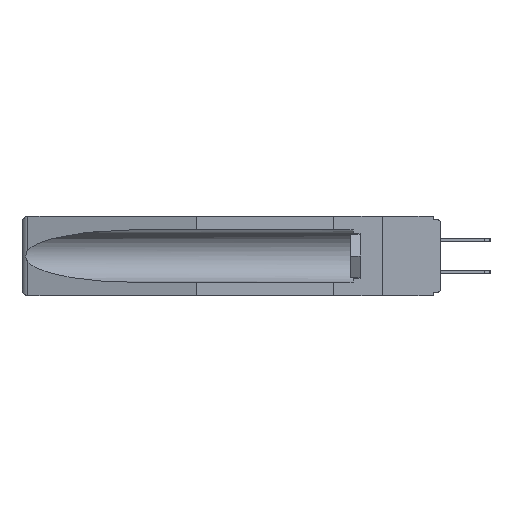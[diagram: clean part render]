
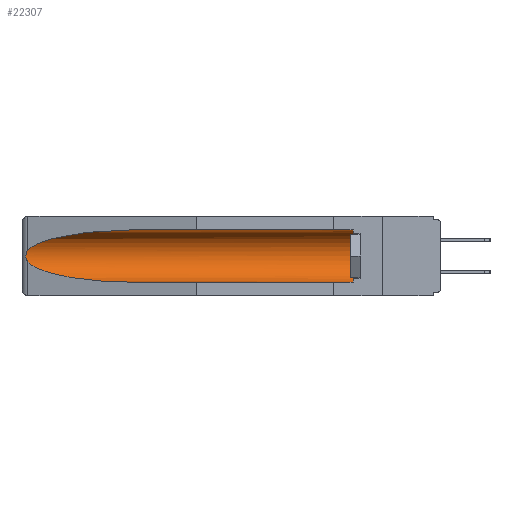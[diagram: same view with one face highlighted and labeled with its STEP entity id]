
A CAD part, left-side view. The second image highlights one B-rep face of the part: STEP entity #22307.
In plain terms, the highlighted cylindrical face has radius 2.857 mm (diameter 5.715 mm), a partial arc.
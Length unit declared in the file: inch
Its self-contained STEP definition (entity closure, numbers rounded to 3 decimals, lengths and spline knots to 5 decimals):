
#1272 = CARTESIAN_POINT ( 'NONE',  ( 0.25451, 1.48313, -0.09465 ) ) ;
#1772 = EDGE_CURVE ( 'NONE', #12204, #23187, #22237, .T. ) ;
#1898 = CARTESIAN_POINT ( 'NONE',  ( 0.26537, 1.52718, -0.14972 ) ) ;
#2437 = VERTEX_POINT ( 'NONE', #14347 ) ;
#3935 = CYLINDRICAL_SURFACE ( 'NONE', #19691, 0.1125 ) ;
#4100 = CARTESIAN_POINT ( 'NONE',  ( 0.2675, 1.53308, -0.17534 ) ) ;
#4671 = VERTEX_POINT ( 'NONE', #19808 ) ;
#5246 = CARTESIAN_POINT ( 'NONE',  ( 0.155, 0.126, -0.284 ) ) ;
#5372 =( BOUNDED_CURVE ( )  B_SPLINE_CURVE ( 3, ( #25111, #15462, #1272, #17284 ),
 .UNSPECIFIED., .F., .F. ) 
 B_SPLINE_CURVE_WITH_KNOTS ( ( 4, 4 ),
 ( 4.71239, 6.08839 ),
 .UNSPECIFIED. ) 
 CURVE ( )  GEOMETRIC_REPRESENTATION_ITEM ( )  RATIONAL_B_SPLINE_CURVE ( ( 1., 0.848, 0.848, 1. ) ) 
 REPRESENTATION_ITEM ( '' )  );
#5469 = VECTOR ( 'NONE', #18364, 39.37008 ) ;
#6264 = DIRECTION ( 'NONE',  ( 0., 0., 1. ) ) ;
#7159 = CARTESIAN_POINT ( 'NONE',  ( 0.26537, 1.52718, -0.19328 ) ) ;
#7236 = B_SPLINE_CURVE_WITH_KNOTS ( 'NONE', 3,
 ( #12720, #18549, #12638, #12551, #15929, #4100, #8487, #8741, #22394, #10460 ),
 .UNSPECIFIED., .F., .F.,
 ( 4, 2, 2, 2, 4 ),
 ( 0., 0.00029, 0.00058, 0.00087, 0.00117 ),
 .UNSPECIFIED. ) ;
#7256 = ORIENTED_EDGE ( 'NONE', *, *, #1772, .T. ) ;
#7600 = CARTESIAN_POINT ( 'NONE',  ( 0.155, 1.07973, -0.284 ) ) ;
#7628 = CARTESIAN_POINT ( 'NONE',  ( 0.155, -0.30754, -0.1715 ) ) ;
#7935 = VERTEX_POINT ( 'NONE', #5246 ) ;
#8487 = CARTESIAN_POINT ( 'NONE',  ( 0.2673, 1.53269, -0.17917 ) ) ;
#8741 = CARTESIAN_POINT ( 'NONE',  ( 0.26655, 1.53094, -0.18657 ) ) ;
#8783 = CARTESIAN_POINT ( 'NONE',  ( 0.26537, 1.52718, -0.19328 ) ) ;
#9243 = VECTOR ( 'NONE', #23481, 39.37008 ) ;
#9621 = DIRECTION ( 'NONE',  ( 0., 0., 1. ) ) ;
#10022 = EDGE_LOOP ( 'NONE', ( #16027, #10318, #7256, #18476, #14307, #12264 ) ) ;
#10318 = ORIENTED_EDGE ( 'NONE', *, *, #20927, .T. ) ;
#10460 = CARTESIAN_POINT ( 'NONE',  ( 0.26537, 1.52718, -0.19328 ) ) ;
#10995 = CARTESIAN_POINT ( 'NONE',  ( 0.155, 1.07973, -0.284 ) ) ;
#11872 = DIRECTION ( 'NONE',  ( 0., -1., 0. ) ) ;
#12204 = VERTEX_POINT ( 'NONE', #7159 ) ;
#12264 = ORIENTED_EDGE ( 'NONE', *, *, #15614, .T. ) ;
#12287 = CARTESIAN_POINT ( 'NONE',  ( 0.155, -0.30754, -0.059 ) ) ;
#12332 = EDGE_CURVE ( 'NONE', #7935, #4671, #13960, .T. ) ;
#12551 = CARTESIAN_POINT ( 'NONE',  ( 0.2673, 1.5327, -0.16383 ) ) ;
#12628 = EDGE_CURVE ( 'NONE', #2437, #24193, #5372, .T. ) ;
#12638 = CARTESIAN_POINT ( 'NONE',  ( 0.26654, 1.53092, -0.15636 ) ) ;
#12720 = CARTESIAN_POINT ( 'NONE',  ( 0.26537, 1.52718, -0.14972 ) ) ;
#13244 = DIRECTION ( 'NONE',  ( 0., 1., 0. ) ) ;
#13813 = FACE_OUTER_BOUND ( 'NONE', #10022, .T. ) ;
#13896 = LINE ( 'NONE', #21568, #9243 ) ;
#13960 = CIRCLE ( 'NONE', #17753, 0.1125 ) ;
#14307 = ORIENTED_EDGE ( 'NONE', *, *, #12332, .T. ) ;
#14347 = CARTESIAN_POINT ( 'NONE',  ( 0.155, 1.07973, -0.059 ) ) ;
#15462 = CARTESIAN_POINT ( 'NONE',  ( 0.21114, 1.30732, -0.059 ) ) ;
#15614 = EDGE_CURVE ( 'NONE', #4671, #2437, #25646, .T. ) ;
#15929 = CARTESIAN_POINT ( 'NONE',  ( 0.2675, 1.53308, -0.16763 ) ) ;
#16027 = ORIENTED_EDGE ( 'NONE', *, *, #12628, .T. ) ;
#16829 = CARTESIAN_POINT ( 'NONE',  ( 0.25451, 1.48313, -0.24835 ) ) ;
#17284 = CARTESIAN_POINT ( 'NONE',  ( 0.26537, 1.52718, -0.14972 ) ) ;
#17753 = AXIS2_PLACEMENT_3D ( 'NONE', #23770, #11872, #6264 ) ;
#18364 = DIRECTION ( 'NONE',  ( 0., 1., 0. ) ) ;
#18476 = ORIENTED_EDGE ( 'NONE', *, *, #24219, .F. ) ;
#18549 = CARTESIAN_POINT ( 'NONE',  ( 0.26597, 1.52961, -0.15275 ) ) ;
#19691 = AXIS2_PLACEMENT_3D ( 'NONE', #7628, #13244, #9621 ) ;
#19808 = CARTESIAN_POINT ( 'NONE',  ( 0.155, 0.126, -0.059 ) ) ;
#20927 = EDGE_CURVE ( 'NONE', #24193, #12204, #7236, .T. ) ;
#21568 = CARTESIAN_POINT ( 'NONE',  ( 0.155, -0.30754, -0.284 ) ) ;
#22237 =( BOUNDED_CURVE ( )  B_SPLINE_CURVE ( 3, ( #8783, #16829, #22687, #10995 ),
 .UNSPECIFIED., .F., .F. ) 
 B_SPLINE_CURVE_WITH_KNOTS ( ( 4, 4 ),
 ( 0.1948, 1.5708 ),
 .UNSPECIFIED. ) 
 CURVE ( )  GEOMETRIC_REPRESENTATION_ITEM ( )  RATIONAL_B_SPLINE_CURVE ( ( 1., 0.848, 0.848, 1. ) ) 
 REPRESENTATION_ITEM ( '' )  );
#22307 = ADVANCED_FACE ( 'NONE', ( #13813 ), #3935, .F. ) ;
#22394 = CARTESIAN_POINT ( 'NONE',  ( 0.26597, 1.5296, -0.19026 ) ) ;
#22687 = CARTESIAN_POINT ( 'NONE',  ( 0.21114, 1.30732, -0.284 ) ) ;
#23187 = VERTEX_POINT ( 'NONE', #7600 ) ;
#23481 = DIRECTION ( 'NONE',  ( 0., 1., 0. ) ) ;
#23770 = CARTESIAN_POINT ( 'NONE',  ( 0.155, 0.126, -0.1715 ) ) ;
#24193 = VERTEX_POINT ( 'NONE', #1898 ) ;
#24219 = EDGE_CURVE ( 'NONE', #7935, #23187, #13896, .T. ) ;
#25111 = CARTESIAN_POINT ( 'NONE',  ( 0.155, 1.07973, -0.059 ) ) ;
#25646 = LINE ( 'NONE', #12287, #5469 ) ;
